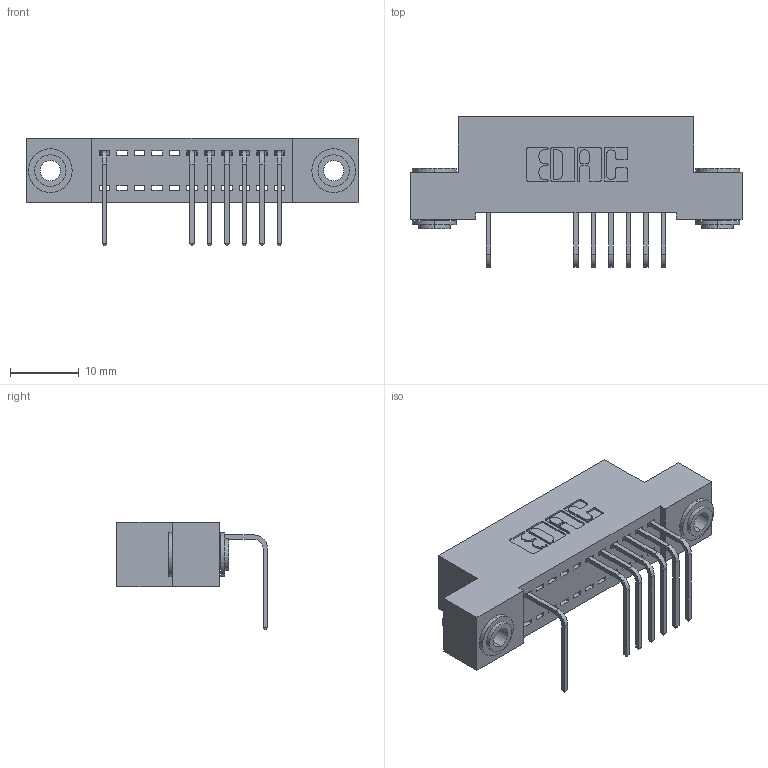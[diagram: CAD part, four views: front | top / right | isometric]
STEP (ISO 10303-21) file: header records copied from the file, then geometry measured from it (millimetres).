
FILE_DESCRIPTION (( 'STEP AP203' ), '1' );
FILE_NAME ('342-011-558-103.STEP', '2018-08-10T14:39:56', ( '' ), ( '' ), 'SwSTEP 2.0', 'SolidWorks 2016', '' );
FILE_SCHEMA (( 'CONFIG_CONTROL_DESIGN' ));
Length unit declared in the file: inch
Products named in the file (4): 345-292-001_558 Tail - 2; 342-250-002_345-250-002-102; 342-011-558-103; 342 Part_.156 TH
Assembly tree (10 placements, depth 2):
  342-011-558-103
    342 Part_.156 TH
    345-292-001_558 Tail - 2  x7
    342-250-002_345-250-002-102  x2
Bounding box: 48.26 x 21.91 x 15.62 mm (x, y, z)
Volume: 4117.7 mm3; surface area: 5589.3 mm2
Topology: 10 solids, 10 shells, 616 faces, 1817 edges, 1198 vertices
Faces by surface type: plane 432, cylinder 176, cone 8
Entity records: 11208 total; most frequent: CARTESIAN_POINT 1934, ORIENTED_EDGE 1878, DIRECTION 1723, EDGE_CURVE 939, VECTOR 787, LINE 787, VERTEX_POINT 622, AXIS2_PLACEMENT_3D 468
